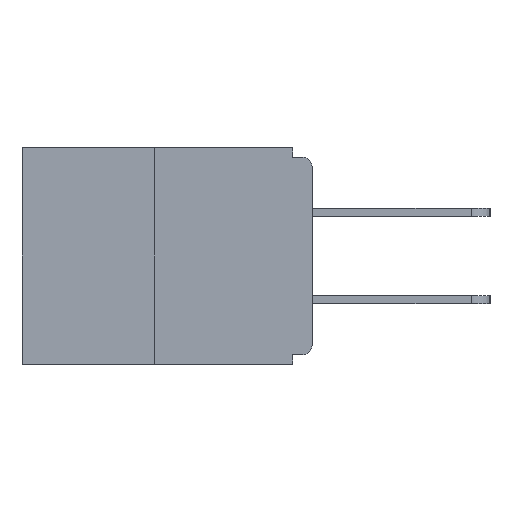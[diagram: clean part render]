
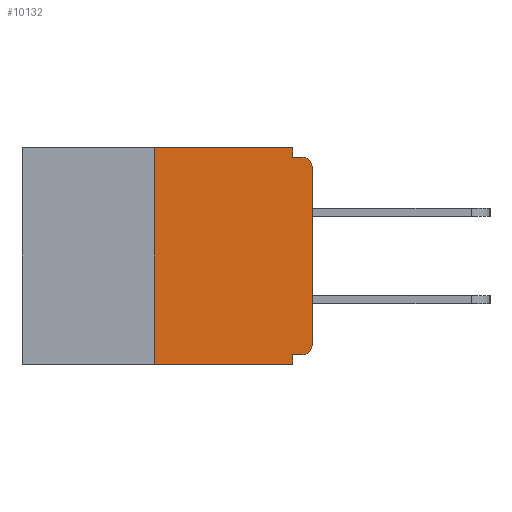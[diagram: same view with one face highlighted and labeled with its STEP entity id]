
A CAD part, left-side view. The second image highlights one B-rep face of the part: STEP entity #10132.
In plain terms, the highlighted planar face has unit normal (-1, 0, 0).
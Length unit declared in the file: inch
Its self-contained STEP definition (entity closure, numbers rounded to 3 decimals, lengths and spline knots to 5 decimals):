
#76 = EDGE_CURVE ( 'NONE', #8517, #4417, #3423, .T. ) ;
#234 = DIRECTION ( 'NONE',  ( 0., 0., -1. ) ) ;
#581 = CARTESIAN_POINT ( 'NONE',  ( 0., 0.46, 0. ) ) ;
#718 = AXIS2_PLACEMENT_3D ( 'NONE', #9212, #7089, #1782 ) ;
#754 = CARTESIAN_POINT ( 'NONE',  ( 0., 0.015, -0.328 ) ) ;
#856 = ORIENTED_EDGE ( 'NONE', *, *, #2021, .F. ) ;
#1242 = VECTOR ( 'NONE', #7722, 39.37008 ) ;
#1499 = EDGE_CURVE ( 'NONE', #12336, #5784, #6887, .T. ) ;
#1692 = VERTEX_POINT ( 'NONE', #4317 ) ;
#1729 = EDGE_CURVE ( 'NONE', #1692, #5784, #5539, .T. ) ;
#1782 = DIRECTION ( 'NONE',  ( 0., 0., -1. ) ) ;
#1796 = CARTESIAN_POINT ( 'NONE',  ( 0., 0.031, -0.343 ) ) ;
#2021 = EDGE_CURVE ( 'NONE', #8263, #12336, #6526, .T. ) ;
#2171 = CARTESIAN_POINT ( 'NONE',  ( 0., 0.031, -0.015 ) ) ;
#2407 = CARTESIAN_POINT ( 'NONE',  ( 0., 0.25, 0. ) ) ;
#2410 = DIRECTION ( 'NONE',  ( 0., 0., 1. ) ) ;
#2620 = ORIENTED_EDGE ( 'NONE', *, *, #4584, .T. ) ;
#2721 = DIRECTION ( 'NONE',  ( 0., 0., -1. ) ) ;
#3098 = CARTESIAN_POINT ( 'NONE',  ( 0., 0.25, -0.343 ) ) ;
#3113 = CARTESIAN_POINT ( 'NONE',  ( 0., 0.031, -0.328 ) ) ;
#3423 = LINE ( 'NONE', #2407, #10370 ) ;
#3455 = CARTESIAN_POINT ( 'NONE',  ( 0., 0.031, 0. ) ) ;
#3499 = CARTESIAN_POINT ( 'NONE',  ( 0., 0.015, -0.03 ) ) ;
#3663 = VECTOR ( 'NONE', #2721, 39.37008 ) ;
#3865 = CARTESIAN_POINT ( 'NONE',  ( 0., 0.031, -0.343 ) ) ;
#3990 = DIRECTION ( 'NONE',  ( 0., 0., -1. ) ) ;
#4317 = CARTESIAN_POINT ( 'NONE',  ( 0., 0., -0.03 ) ) ;
#4417 = VERTEX_POINT ( 'NONE', #5412 ) ;
#4546 = CARTESIAN_POINT ( 'NONE',  ( 0., 0., -0.015 ) ) ;
#4584 = EDGE_CURVE ( 'NONE', #12958, #1692, #9843, .T. ) ;
#4832 = ORIENTED_EDGE ( 'NONE', *, *, #7611, .F. ) ;
#4874 = VERTEX_POINT ( 'NONE', #1796 ) ;
#5052 = CARTESIAN_POINT ( 'NONE',  ( 0., 0.031, 0. ) ) ;
#5206 = ORIENTED_EDGE ( 'NONE', *, *, #1499, .F. ) ;
#5309 = LINE ( 'NONE', #3865, #5984 ) ;
#5412 = CARTESIAN_POINT ( 'NONE',  ( 0., 0.25, 0. ) ) ;
#5539 = CIRCLE ( 'NONE', #11081, 0.015 ) ;
#5651 = CARTESIAN_POINT ( 'NONE',  ( 0., 0., 0. ) ) ;
#5692 = EDGE_CURVE ( 'NONE', #8517, #4874, #9473, .T. ) ;
#5784 = VERTEX_POINT ( 'NONE', #7874 ) ;
#5796 = CARTESIAN_POINT ( 'NONE',  ( 0., 0.46, -0.343 ) ) ;
#5984 = VECTOR ( 'NONE', #7165, 39.37008 ) ;
#6526 = LINE ( 'NONE', #5052, #3663 ) ;
#6594 = VECTOR ( 'NONE', #10155, 39.37008 ) ;
#6662 = LINE ( 'NONE', #12101, #1242 ) ;
#6667 = ORIENTED_EDGE ( 'NONE', *, *, #9093, .F. ) ;
#6816 = EDGE_CURVE ( 'NONE', #10148, #9315, #6662, .T. ) ;
#6887 = LINE ( 'NONE', #4546, #12822 ) ;
#7089 = DIRECTION ( 'NONE',  ( -1., 0., 0. ) ) ;
#7165 = DIRECTION ( 'NONE',  ( 0., 0., -1. ) ) ;
#7294 = ORIENTED_EDGE ( 'NONE', *, *, #6816, .F. ) ;
#7611 = EDGE_CURVE ( 'NONE', #9315, #4874, #5309, .T. ) ;
#7696 = DIRECTION ( 'NONE',  ( 0., -1., 0. ) ) ;
#7722 = DIRECTION ( 'NONE',  ( 0., 1., 0. ) ) ;
#7874 = CARTESIAN_POINT ( 'NONE',  ( 0., 0.015, -0.015 ) ) ;
#8263 = VERTEX_POINT ( 'NONE', #3455 ) ;
#8374 = PLANE ( 'NONE',  #13835 ) ;
#8455 = DIRECTION ( 'NONE',  ( 1., 0., 0. ) ) ;
#8517 = VERTEX_POINT ( 'NONE', #3098 ) ;
#9093 = EDGE_CURVE ( 'NONE', #4417, #8263, #13381, .T. ) ;
#9212 = CARTESIAN_POINT ( 'NONE',  ( 0., 0.015, -0.313 ) ) ;
#9315 = VERTEX_POINT ( 'NONE', #3113 ) ;
#9473 = LINE ( 'NONE', #5796, #6594 ) ;
#9808 = ORIENTED_EDGE ( 'NONE', *, *, #13653, .T. ) ;
#9843 = LINE ( 'NONE', #5651, #12403 ) ;
#10132 = ADVANCED_FACE ( 'NONE', ( #11475 ), #8374, .F. ) ;
#10148 = VERTEX_POINT ( 'NONE', #754 ) ;
#10155 = DIRECTION ( 'NONE',  ( 0., -1., 0. ) ) ;
#10287 = DIRECTION ( 'NONE',  ( 0., -1., 0. ) ) ;
#10370 = VECTOR ( 'NONE', #11208, 39.37008 ) ;
#11081 = AXIS2_PLACEMENT_3D ( 'NONE', #3499, #11975, #234 ) ;
#11208 = DIRECTION ( 'NONE',  ( 0., 0., 1. ) ) ;
#11475 = FACE_OUTER_BOUND ( 'NONE', #12245, .T. ) ;
#11975 = DIRECTION ( 'NONE',  ( -1., 0., 0. ) ) ;
#12101 = CARTESIAN_POINT ( 'NONE',  ( 0., 0., -0.328 ) ) ;
#12245 = EDGE_LOOP ( 'NONE', ( #6667, #12593, #13842, #4832, #7294, #9808, #2620, #12743, #5206, #856 ) ) ;
#12279 = CARTESIAN_POINT ( 'NONE',  ( 0., 0., -0.313 ) ) ;
#12336 = VERTEX_POINT ( 'NONE', #2171 ) ;
#12403 = VECTOR ( 'NONE', #2410, 39.37008 ) ;
#12593 = ORIENTED_EDGE ( 'NONE', *, *, #76, .F. ) ;
#12603 = CARTESIAN_POINT ( 'NONE',  ( 0., 0.46, 0. ) ) ;
#12707 = VECTOR ( 'NONE', #10287, 39.37008 ) ;
#12743 = ORIENTED_EDGE ( 'NONE', *, *, #1729, .T. ) ;
#12822 = VECTOR ( 'NONE', #7696, 39.37008 ) ;
#12935 = CIRCLE ( 'NONE', #718, 0.015 ) ;
#12958 = VERTEX_POINT ( 'NONE', #12279 ) ;
#13381 = LINE ( 'NONE', #581, #12707 ) ;
#13653 = EDGE_CURVE ( 'NONE', #10148, #12958, #12935, .T. ) ;
#13835 = AXIS2_PLACEMENT_3D ( 'NONE', #12603, #8455, #3990 ) ;
#13842 = ORIENTED_EDGE ( 'NONE', *, *, #5692, .T. ) ;
